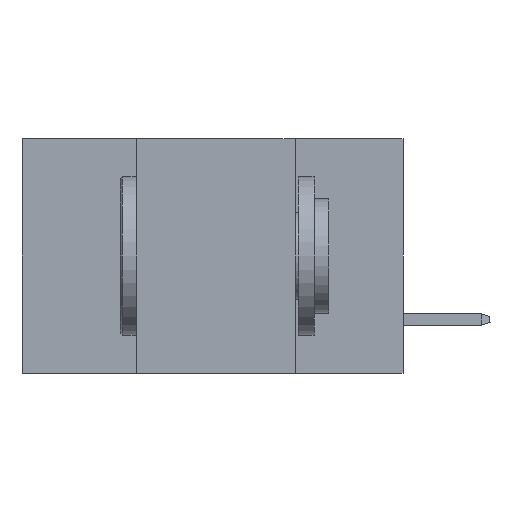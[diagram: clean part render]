
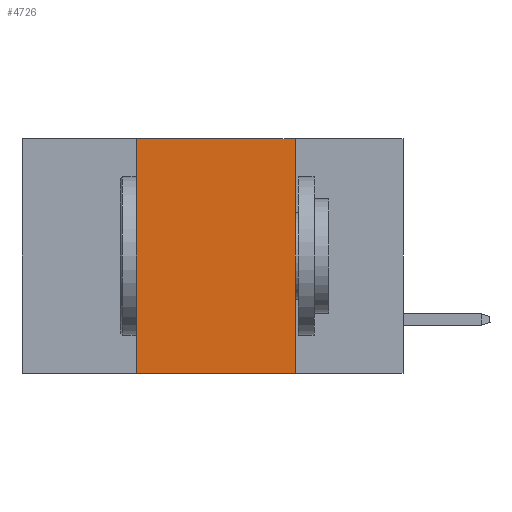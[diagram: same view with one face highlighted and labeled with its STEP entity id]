
A CAD part, left-side view. The second image highlights one B-rep face of the part: STEP entity #4726.
In plain terms, the highlighted planar face has unit normal (-1, 0, 0).
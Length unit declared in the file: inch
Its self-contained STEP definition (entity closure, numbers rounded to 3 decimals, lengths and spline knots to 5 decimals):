
#1147 = VERTEX_POINT ( 'NONE', #13069 ) ;
#1935 = PLANE ( 'NONE',  #15313 ) ;
#2287 = FACE_OUTER_BOUND ( 'NONE', #4637, .T. ) ;
#2389 = VERTEX_POINT ( 'NONE', #22253 ) ;
#2588 = ORIENTED_EDGE ( 'NONE', *, *, #22255, .F. ) ;
#3733 = DIRECTION ( 'NONE',  ( 0., 0., -1. ) ) ;
#4637 = EDGE_LOOP ( 'NONE', ( #2588, #6110, #15107, #11944 ) ) ;
#4726 = ADVANCED_FACE ( 'NONE', ( #2287 ), #1935, .F. ) ;
#5510 = DIRECTION ( 'NONE',  ( 1., 0., 0. ) ) ;
#6110 = ORIENTED_EDGE ( 'NONE', *, *, #15466, .F. ) ;
#6376 = LINE ( 'NONE', #11713, #22971 ) ;
#7210 = LINE ( 'NONE', #14745, #21070 ) ;
#7758 = DIRECTION ( 'NONE',  ( 0., -1., 0. ) ) ;
#8694 = CARTESIAN_POINT ( 'NONE',  ( 0., 0.42, -0.37 ) ) ;
#9077 = DIRECTION ( 'NONE',  ( 0., 0., 1. ) ) ;
#11713 = CARTESIAN_POINT ( 'NONE',  ( 0., 0.6, 0. ) ) ;
#11944 = ORIENTED_EDGE ( 'NONE', *, *, #17428, .T. ) ;
#13069 = CARTESIAN_POINT ( 'NONE',  ( 0., 0.42, 0. ) ) ;
#13129 = LINE ( 'NONE', #20666, #19206 ) ;
#13441 = LINE ( 'NONE', #20976, #20209 ) ;
#13534 = CARTESIAN_POINT ( 'NONE',  ( 0., 0.6, 0. ) ) ;
#13923 = DIRECTION ( 'NONE',  ( 0., -1., 0. ) ) ;
#14745 = CARTESIAN_POINT ( 'NONE',  ( 0., 0.42, 0. ) ) ;
#15107 = ORIENTED_EDGE ( 'NONE', *, *, #19333, .F. ) ;
#15313 = AXIS2_PLACEMENT_3D ( 'NONE', #13534, #5510, #18985 ) ;
#15466 = EDGE_CURVE ( 'NONE', #1147, #2389, #6376, .T. ) ;
#17428 = EDGE_CURVE ( 'NONE', #22093, #22973, #13441, .T. ) ;
#18985 = DIRECTION ( 'NONE',  ( 0., 0., -1. ) ) ;
#19206 = VECTOR ( 'NONE', #3733, 39.37008 ) ;
#19333 = EDGE_CURVE ( 'NONE', #22093, #1147, #7210, .T. ) ;
#19634 = CARTESIAN_POINT ( 'NONE',  ( 0., 0.17, -0.37 ) ) ;
#20209 = VECTOR ( 'NONE', #7758, 39.37008 ) ;
#20666 = CARTESIAN_POINT ( 'NONE',  ( 0., 0.17, 0. ) ) ;
#20976 = CARTESIAN_POINT ( 'NONE',  ( 0., 0.6, -0.37 ) ) ;
#21070 = VECTOR ( 'NONE', #9077, 39.37008 ) ;
#22093 = VERTEX_POINT ( 'NONE', #8694 ) ;
#22253 = CARTESIAN_POINT ( 'NONE',  ( 0., 0.17, 0. ) ) ;
#22255 = EDGE_CURVE ( 'NONE', #2389, #22973, #13129, .T. ) ;
#22971 = VECTOR ( 'NONE', #13923, 39.37008 ) ;
#22973 = VERTEX_POINT ( 'NONE', #19634 ) ;
